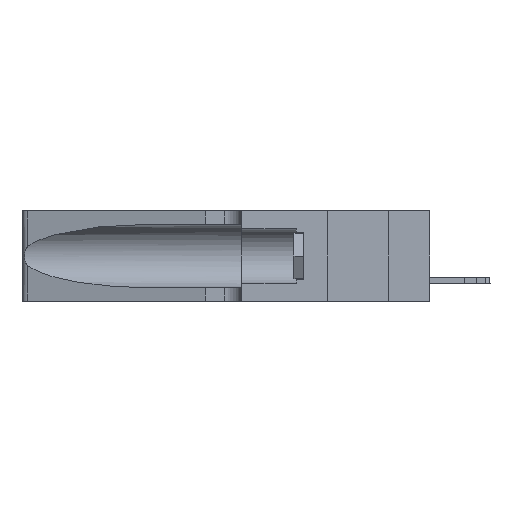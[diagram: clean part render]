
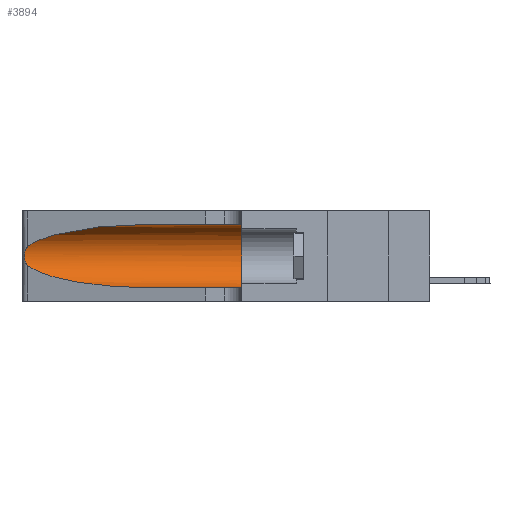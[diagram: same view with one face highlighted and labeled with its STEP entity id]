
A CAD part, left-side view. The second image highlights one B-rep face of the part: STEP entity #3894.
In plain terms, the highlighted cylindrical face has radius 3.308 mm (diameter 6.617 mm), a partial arc.
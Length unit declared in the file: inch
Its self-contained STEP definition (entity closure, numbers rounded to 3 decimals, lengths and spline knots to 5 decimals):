
#1418 = CARTESIAN_POINT ( 'NONE',  ( 0.18966, 0.96281, 0.05475 ) ) ;
#1603 = CARTESIAN_POINT ( 'NONE',  ( 0.25787, 1.23484, 0.2124 ) ) ;
#1767 = CARTESIAN_POINT ( 'NONE',  ( 0.26075, 1.23896, 0.19203 ) ) ;
#2584 = AXIS2_PLACEMENT_3D ( 'NONE', #12016, #15970, #19808 ) ;
#3308 = EDGE_CURVE ( 'NONE', #10117, #22812, #13623, .T. ) ;
#3455 = ORIENTED_EDGE ( 'NONE', *, *, #3308, .F. ) ;
#3659 = CARTESIAN_POINT ( 'NONE',  ( 0.25639, 1.23186, 0.15144 ) ) ;
#3873 = DIRECTION ( 'NONE',  ( 0., 0., -1. ) ) ;
#3894 = ADVANCED_FACE ( 'NONE', ( #15739 ), #24434, .F. ) ;
#4116 = VERTEX_POINT ( 'NONE', #18553 ) ;
#4160 = EDGE_CURVE ( 'NONE', #19620, #22600, #18126, .T. ) ;
#4880 = VECTOR ( 'NONE', #14873, 39.37008 ) ;
#5169 = VERTEX_POINT ( 'NONE', #9746 ) ;
#5237 = ORIENTED_EDGE ( 'NONE', *, *, #4160, .T. ) ;
#5531 = CARTESIAN_POINT ( 'NONE',  ( 0.25789, 1.23486, 0.15765 ) ) ;
#5792 = CARTESIAN_POINT ( 'NONE',  ( 0.25856, 1.23593, 0.16098 ) ) ;
#5961 = CARTESIAN_POINT ( 'NONE',  ( 0.1305, 1.61858, 0.31525 ) ) ;
#6185 = CARTESIAN_POINT ( 'NONE',  ( 0.18966, 0.96281, 0.31525 ) ) ;
#6349 = CARTESIAN_POINT ( 'NONE',  ( 0.1305, 0.72297, 0.31525 ) ) ;
#7355 = CARTESIAN_POINT ( 'NONE',  ( 0.25487, 1.22718, 0.22369 ) ) ;
#7382 = AXIS2_PLACEMENT_3D ( 'NONE', #15605, #19473, #3873 ) ;
#8830 = EDGE_CURVE ( 'NONE', #4116, #19620, #17086, .T. ) ;
#9413 = CARTESIAN_POINT ( 'NONE',  ( 0.25555, 1.22993, 0.14849 ) ) ;
#9627 = CARTESIAN_POINT ( 'NONE',  ( 0.1305, 1.61858, 0.05475 ) ) ;
#9689 = CARTESIAN_POINT ( 'NONE',  ( 0.25487, 1.22718, 0.14631 ) ) ;
#9746 = CARTESIAN_POINT ( 'NONE',  ( 0.1305, 0.35, 0.05475 ) ) ;
#10105 = LINE ( 'NONE', #9627, #4880 ) ;
#10117 = VERTEX_POINT ( 'NONE', #14299 ) ;
#11183 = CARTESIAN_POINT ( 'NONE',  ( 0.25487, 1.22718, 0.14631 ) ) ;
#11268 = CARTESIAN_POINT ( 'NONE',  ( 0.1305, 0.72297, 0.05475 ) ) ;
#11441 = CARTESIAN_POINT ( 'NONE',  ( 0.25854, 1.2359, 0.20912 ) ) ;
#11519 = CARTESIAN_POINT ( 'NONE',  ( 0.26075, 1.23896, 0.178 ) ) ;
#12004 = EDGE_CURVE ( 'NONE', #22600, #5169, #10105, .T. ) ;
#12016 = CARTESIAN_POINT ( 'NONE',  ( 0.1305, 0.35, 0.185 ) ) ;
#12359 = CARTESIAN_POINT ( 'NONE',  ( 0.25487, 1.22718, 0.14631 ) ) ;
#13449 = EDGE_CURVE ( 'NONE', #10117, #4116, #16176, .T. ) ;
#13577 = CARTESIAN_POINT ( 'NONE',  ( 0.25639, 1.23184, 0.21858 ) ) ;
#13623 = LINE ( 'NONE', #5961, #17563 ) ;
#14021 = CARTESIAN_POINT ( 'NONE',  ( 0.2373, 1.15595, 0.28018 ) ) ;
#14299 = CARTESIAN_POINT ( 'NONE',  ( 0.1305, 0.72297, 0.31525 ) ) ;
#14873 = DIRECTION ( 'NONE',  ( 0., -1., 0. ) ) ;
#15605 = CARTESIAN_POINT ( 'NONE',  ( 0.1305, 1.61858, 0.185 ) ) ;
#15739 = FACE_OUTER_BOUND ( 'NONE', #19871, .T. ) ;
#15873 = ORIENTED_EDGE ( 'NONE', *, *, #12004, .T. ) ;
#15970 = DIRECTION ( 'NONE',  ( 0., 1., 0. ) ) ;
#16176 =( BOUNDED_CURVE ( )  B_SPLINE_CURVE ( 3, ( #6349, #6185, #14021, #23884 ),
 .UNSPECIFIED., .F., .F. ) 
 B_SPLINE_CURVE_WITH_KNOTS ( ( 4, 4 ),
 ( 1.5708, 2.84003 ),
 .UNSPECIFIED. ) 
 CURVE ( )  GEOMETRIC_REPRESENTATION_ITEM ( )  RATIONAL_B_SPLINE_CURVE ( ( 1., 0.87, 0.87, 1. ) ) 
 REPRESENTATION_ITEM ( '' )  );
#17086 = B_SPLINE_CURVE_WITH_KNOTS ( 'NONE', 3,
 ( #7355, #21174, #13577, #1603, #11441, #19075, #1767, #11519, #21005, #5792, #5531, #3659, #9413, #9689 ),
 .UNSPECIFIED., .F., .F.,
 ( 4, 2, 2, 2, 2, 2, 4 ),
 ( 0., 0.00027, 0.00053, 0.00107, 0.0016, 0.00187, 0.00214 ),
 .UNSPECIFIED. ) ;
#17280 = CARTESIAN_POINT ( 'NONE',  ( 0.1305, 0.35, 0.31525 ) ) ;
#17563 = VECTOR ( 'NONE', #23586, 39.37008 ) ;
#18126 =( BOUNDED_CURVE ( )  B_SPLINE_CURVE ( 3, ( #11183, #22680, #1418, #11268 ),
 .UNSPECIFIED., .F., .F. ) 
 B_SPLINE_CURVE_WITH_KNOTS ( ( 4, 4 ),
 ( 3.44316, 4.71239 ),
 .UNSPECIFIED. ) 
 CURVE ( )  GEOMETRIC_REPRESENTATION_ITEM ( )  RATIONAL_B_SPLINE_CURVE ( ( 1., 0.87, 0.87, 1. ) ) 
 REPRESENTATION_ITEM ( '' )  );
#18553 = CARTESIAN_POINT ( 'NONE',  ( 0.25487, 1.22718, 0.22369 ) ) ;
#19047 = EDGE_CURVE ( 'NONE', #22812, #5169, #24877, .T. ) ;
#19075 = CARTESIAN_POINT ( 'NONE',  ( 0.26018, 1.23835, 0.19895 ) ) ;
#19313 = ORIENTED_EDGE ( 'NONE', *, *, #8830, .T. ) ;
#19473 = DIRECTION ( 'NONE',  ( 0., -1., 0. ) ) ;
#19620 = VERTEX_POINT ( 'NONE', #12359 ) ;
#19808 = DIRECTION ( 'NONE',  ( 0., 0., 1. ) ) ;
#19871 = EDGE_LOOP ( 'NONE', ( #20872, #19313, #5237, #15873, #21795, #3455 ) ) ;
#20872 = ORIENTED_EDGE ( 'NONE', *, *, #13449, .T. ) ;
#21005 = CARTESIAN_POINT ( 'NONE',  ( 0.26017, 1.23833, 0.17102 ) ) ;
#21174 = CARTESIAN_POINT ( 'NONE',  ( 0.25555, 1.22994, 0.2215 ) ) ;
#21795 = ORIENTED_EDGE ( 'NONE', *, *, #19047, .F. ) ;
#22600 = VERTEX_POINT ( 'NONE', #23975 ) ;
#22680 = CARTESIAN_POINT ( 'NONE',  ( 0.2373, 1.15595, 0.08982 ) ) ;
#22812 = VERTEX_POINT ( 'NONE', #17280 ) ;
#23586 = DIRECTION ( 'NONE',  ( 0., -1., 0. ) ) ;
#23884 = CARTESIAN_POINT ( 'NONE',  ( 0.25487, 1.22718, 0.22369 ) ) ;
#23975 = CARTESIAN_POINT ( 'NONE',  ( 0.1305, 0.72297, 0.05475 ) ) ;
#24434 = CYLINDRICAL_SURFACE ( 'NONE', #7382, 0.13025 ) ;
#24877 = CIRCLE ( 'NONE', #2584, 0.13025 ) ;
